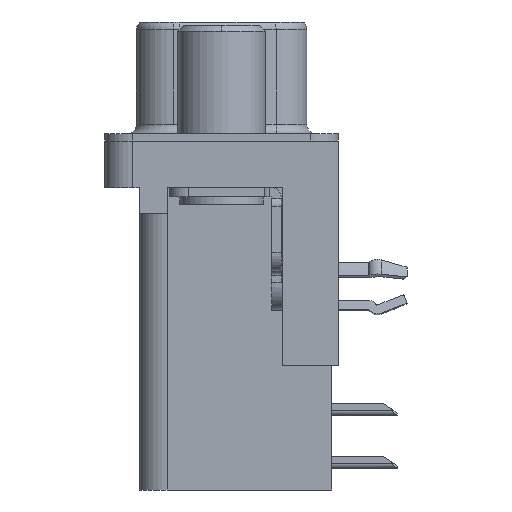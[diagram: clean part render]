
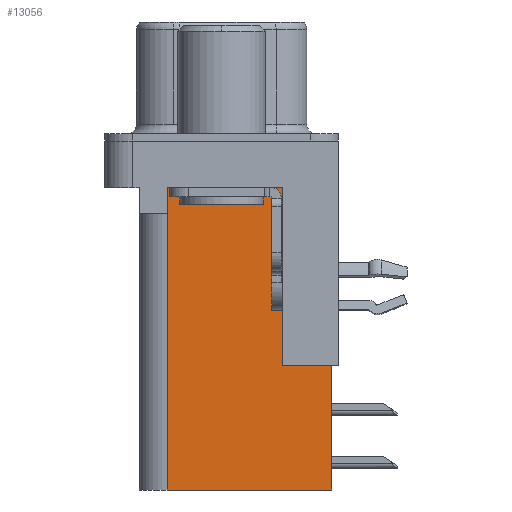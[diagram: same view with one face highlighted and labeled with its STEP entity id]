
A CAD part, left-side view. The second image highlights one B-rep face of the part: STEP entity #13056.
In plain terms, the highlighted planar face has unit normal (-1, 0, 0).
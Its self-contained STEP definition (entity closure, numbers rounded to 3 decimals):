
#21 = EDGE_LOOP ( 'NONE', ( #15708, #7827, #5438, #14865, #423, #15615, #11160, #16330 ) ) ;
#125 = CARTESIAN_POINT ( 'NONE',  ( 3.765, 2.925, -3.9 ) ) ;
#301 = CARTESIAN_POINT ( 'NONE',  ( 3.765, 2.895, -3.9 ) ) ;
#423 = ORIENTED_EDGE ( 'NONE', *, *, #6759, .F. ) ;
#780 = CARTESIAN_POINT ( 'NONE',  ( 3.765, 2.925, -18.76 ) ) ;
#1050 = DIRECTION ( 'NONE',  ( 0., 1., 0. ) ) ;
#1155 = CARTESIAN_POINT ( 'NONE',  ( 3.765, -3.295, -12.05 ) ) ;
#1285 = VERTEX_POINT ( 'NONE', #16012 ) ;
#1987 = FACE_OUTER_BOUND ( 'NONE', #21, .T. ) ;
#2174 = DIRECTION ( 'NONE',  ( 0., 1., 0. ) ) ;
#3305 = CARTESIAN_POINT ( 'NONE',  ( 3.765, -5.925, -2. ) ) ;
#3557 = EDGE_CURVE ( 'NONE', #1285, #12248, #20228, .T. ) ;
#3591 = VECTOR ( 'NONE', #20552, 1000. ) ;
#4290 = CARTESIAN_POINT ( 'NONE',  ( 3.765, -5.925, -18.76 ) ) ;
#4416 = CARTESIAN_POINT ( 'NONE',  ( 3.765, -6.295, -12.05 ) ) ;
#4538 = CARTESIAN_POINT ( 'NONE',  ( 3.765, -3.295, -2.5 ) ) ;
#4980 = LINE ( 'NONE', #20653, #5477 ) ;
#5067 = PLANE ( 'NONE',  #14390 ) ;
#5172 = EDGE_CURVE ( 'NONE', #1285, #8350, #18138, .T. ) ;
#5438 = ORIENTED_EDGE ( 'NONE', *, *, #8558, .T. ) ;
#5477 = VECTOR ( 'NONE', #10973, 1000. ) ;
#5608 = DIRECTION ( 'NONE',  ( 0., 0., -1. ) ) ;
#6759 = EDGE_CURVE ( 'NONE', #8350, #12533, #17378, .T. ) ;
#7149 = CARTESIAN_POINT ( 'NONE',  ( 3.765, 2.895, -3.9 ) ) ;
#7249 = VECTOR ( 'NONE', #18542, 1000. ) ;
#7724 = EDGE_CURVE ( 'NONE', #12248, #14119, #4980, .T. ) ;
#7827 = ORIENTED_EDGE ( 'NONE', *, *, #12070, .T. ) ;
#8126 = VECTOR ( 'NONE', #5608, 1000. ) ;
#8350 = VERTEX_POINT ( 'NONE', #4290 ) ;
#8451 = CARTESIAN_POINT ( 'NONE',  ( 3.765, -3.295, -18.76 ) ) ;
#8558 = EDGE_CURVE ( 'NONE', #16319, #19450, #13243, .T. ) ;
#8816 = VECTOR ( 'NONE', #1050, 1000. ) ;
#8976 = VECTOR ( 'NONE', #2174, 1000. ) ;
#9943 = DIRECTION ( 'NONE',  ( 0., 1., 0. ) ) ;
#10037 = DIRECTION ( 'NONE',  ( 0., 1., 0. ) ) ;
#10973 = DIRECTION ( 'NONE',  ( 0., 0., 1. ) ) ;
#11160 = ORIENTED_EDGE ( 'NONE', *, *, #3557, .T. ) ;
#12005 = LINE ( 'NONE', #780, #7249 ) ;
#12070 = EDGE_CURVE ( 'NONE', #19441, #16319, #12375, .T. ) ;
#12248 = VERTEX_POINT ( 'NONE', #1155 ) ;
#12299 = CARTESIAN_POINT ( 'NONE',  ( 3.765, -3.295, -18.76 ) ) ;
#12375 = LINE ( 'NONE', #7149, #8126 ) ;
#12533 = VERTEX_POINT ( 'NONE', #13444 ) ;
#13056 = ADVANCED_FACE ( 'NONE', ( #1987 ), #5067, .F. ) ;
#13243 = LINE ( 'NONE', #16459, #17065 ) ;
#13423 = CARTESIAN_POINT ( 'NONE',  ( 3.765, -3.295, -2.5 ) ) ;
#13444 = CARTESIAN_POINT ( 'NONE',  ( 3.765, 2.925, -18.76 ) ) ;
#13854 = VECTOR ( 'NONE', #14567, 1000. ) ;
#13924 = EDGE_CURVE ( 'NONE', #12533, #19450, #12005, .T. ) ;
#14119 = VERTEX_POINT ( 'NONE', #4538 ) ;
#14390 = AXIS2_PLACEMENT_3D ( 'NONE', #8451, #19687, #10037 ) ;
#14567 = DIRECTION ( 'NONE',  ( 0., 0., -1. ) ) ;
#14865 = ORIENTED_EDGE ( 'NONE', *, *, #13924, .F. ) ;
#15615 = ORIENTED_EDGE ( 'NONE', *, *, #5172, .F. ) ;
#15657 = EDGE_CURVE ( 'NONE', #14119, #19441, #17532, .T. ) ;
#15708 = ORIENTED_EDGE ( 'NONE', *, *, #15657, .T. ) ;
#16012 = CARTESIAN_POINT ( 'NONE',  ( 3.765, -5.925, -12.05 ) ) ;
#16319 = VERTEX_POINT ( 'NONE', #301 ) ;
#16330 = ORIENTED_EDGE ( 'NONE', *, *, #7724, .T. ) ;
#16459 = CARTESIAN_POINT ( 'NONE',  ( 3.765, 0., -3.9 ) ) ;
#17065 = VECTOR ( 'NONE', #9943, 1000. ) ;
#17378 = LINE ( 'NONE', #12299, #8816 ) ;
#17532 = LINE ( 'NONE', #13423, #8976 ) ;
#17827 = CARTESIAN_POINT ( 'NONE',  ( 3.765, 2.895, -2.5 ) ) ;
#18138 = LINE ( 'NONE', #3305, #13854 ) ;
#18542 = DIRECTION ( 'NONE',  ( 0., 0., 1. ) ) ;
#19441 = VERTEX_POINT ( 'NONE', #17827 ) ;
#19450 = VERTEX_POINT ( 'NONE', #125 ) ;
#19687 = DIRECTION ( 'NONE',  ( 1., 0., 0. ) ) ;
#20228 = LINE ( 'NONE', #4416, #3591 ) ;
#20552 = DIRECTION ( 'NONE',  ( 0., 1., 0. ) ) ;
#20653 = CARTESIAN_POINT ( 'NONE',  ( 3.765, -3.295, -18.76 ) ) ;
